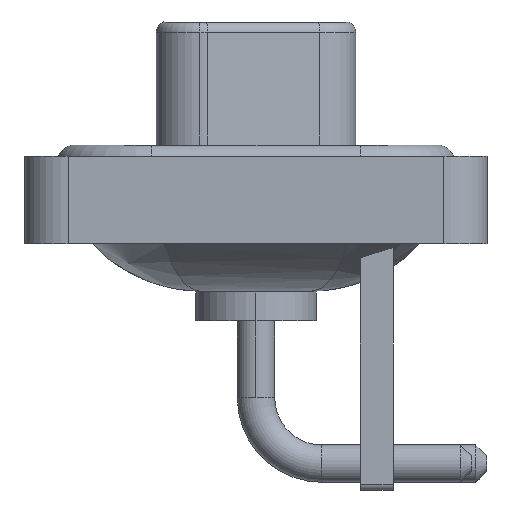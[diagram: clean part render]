
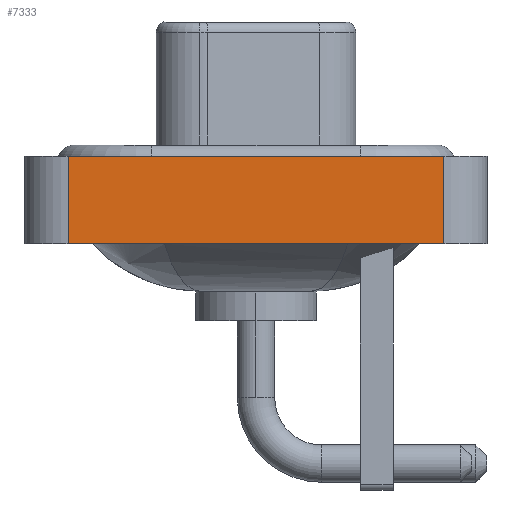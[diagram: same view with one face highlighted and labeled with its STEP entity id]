
A CAD part, left-side view. The second image highlights one B-rep face of the part: STEP entity #7333.
In plain terms, the highlighted planar face has unit normal (-1, 0, 0).
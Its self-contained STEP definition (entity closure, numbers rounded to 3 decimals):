
#588 = DIRECTION ( 'NONE',  ( 0., 0., 1. ) ) ;
#862 = VERTEX_POINT ( 'NONE', #8095 ) ;
#1728 = VECTOR ( 'NONE', #14114, 1000. ) ;
#2600 = EDGE_CURVE ( 'NONE', #12513, #7123, #8848, .T. ) ;
#3818 = PLANE ( 'NONE',  #18541 ) ;
#3890 = LINE ( 'NONE', #14652, #19424 ) ;
#4182 = DIRECTION ( 'NONE',  ( 0., -1., 0. ) ) ;
#4390 = ORIENTED_EDGE ( 'NONE', *, *, #9008, .T. ) ;
#5575 = DIRECTION ( 'NONE',  ( 0., -1., 0. ) ) ;
#7123 = VERTEX_POINT ( 'NONE', #7888 ) ;
#7333 = ADVANCED_FACE ( 'NONE', ( #14574 ), #3818, .T. ) ;
#7855 = EDGE_CURVE ( 'NONE', #862, #7123, #3890, .T. ) ;
#7888 = CARTESIAN_POINT ( 'NONE',  ( -7.3, -8.55, 0.4 ) ) ;
#7965 = CARTESIAN_POINT ( 'NONE',  ( -7.3, 8.55, -3.6 ) ) ;
#8095 = CARTESIAN_POINT ( 'NONE',  ( -7.3, -8.55, -3.6 ) ) ;
#8289 = DIRECTION ( 'NONE',  ( -1., 0., 0. ) ) ;
#8848 = LINE ( 'NONE', #15046, #15839 ) ;
#9008 = EDGE_CURVE ( 'NONE', #16504, #862, #19694, .T. ) ;
#11139 = CARTESIAN_POINT ( 'NONE',  ( -7.3, 8.55, 0.4 ) ) ;
#12185 = ORIENTED_EDGE ( 'NONE', *, *, #7855, .T. ) ;
#12513 = VERTEX_POINT ( 'NONE', #11139 ) ;
#13026 = EDGE_CURVE ( 'NONE', #16504, #12513, #14213, .T. ) ;
#13204 = CARTESIAN_POINT ( 'NONE',  ( -7.3, -8.55, -3.6 ) ) ;
#13718 = ORIENTED_EDGE ( 'NONE', *, *, #2600, .F. ) ;
#14114 = DIRECTION ( 'NONE',  ( 0., 0., 1. ) ) ;
#14213 = LINE ( 'NONE', #16948, #1728 ) ;
#14574 = FACE_OUTER_BOUND ( 'NONE', #17153, .T. ) ;
#14652 = CARTESIAN_POINT ( 'NONE',  ( -7.3, -8.55, -3.6 ) ) ;
#14752 = ORIENTED_EDGE ( 'NONE', *, *, #13026, .F. ) ;
#15046 = CARTESIAN_POINT ( 'NONE',  ( -7.3, -8.55, 0.4 ) ) ;
#15801 = CARTESIAN_POINT ( 'NONE',  ( -7.3, -8.55, -3.6 ) ) ;
#15839 = VECTOR ( 'NONE', #4182, 1000. ) ;
#16504 = VERTEX_POINT ( 'NONE', #7965 ) ;
#16948 = CARTESIAN_POINT ( 'NONE',  ( -7.3, 8.55, -3.6 ) ) ;
#17153 = EDGE_LOOP ( 'NONE', ( #12185, #13718, #14752, #4390 ) ) ;
#18541 = AXIS2_PLACEMENT_3D ( 'NONE', #15801, #8289, #588 ) ;
#19120 = VECTOR ( 'NONE', #5575, 1000. ) ;
#19424 = VECTOR ( 'NONE', #19640, 1000. ) ;
#19640 = DIRECTION ( 'NONE',  ( 0., 0., 1. ) ) ;
#19694 = LINE ( 'NONE', #13204, #19120 ) ;
